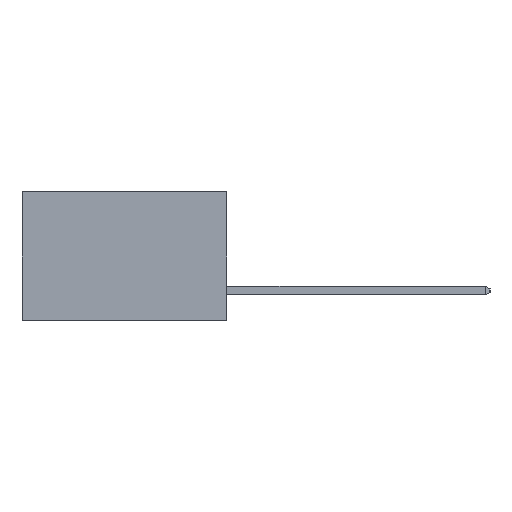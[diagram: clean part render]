
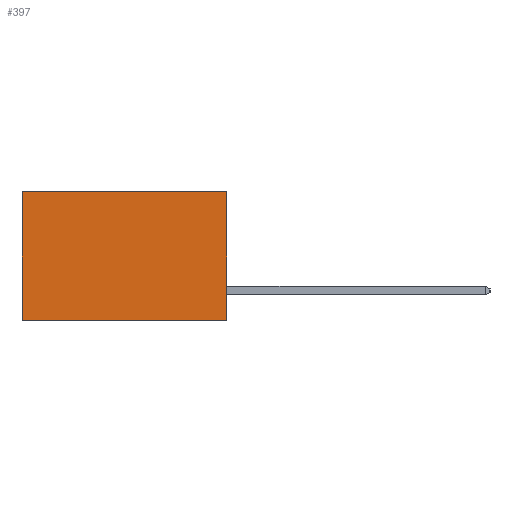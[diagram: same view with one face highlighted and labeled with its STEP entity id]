
A CAD part, left-side view. The second image highlights one B-rep face of the part: STEP entity #397.
In plain terms, the highlighted planar face has unit normal (-1, 0, 0).
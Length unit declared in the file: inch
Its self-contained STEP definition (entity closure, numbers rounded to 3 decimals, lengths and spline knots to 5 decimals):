
#125 = DIRECTION ( 'NONE',  ( 1., 0., 0. ) ) ;
#236 = PLANE ( 'NONE',  #12208 ) ;
#397 = ADVANCED_FACE ( 'NONE', ( #10097 ), #236, .F. ) ;
#1538 = LINE ( 'NONE', #20694, #6214 ) ;
#2117 = VERTEX_POINT ( 'NONE', #7028 ) ;
#2298 = DIRECTION ( 'NONE',  ( 0., 1., 0. ) ) ;
#2622 = EDGE_CURVE ( 'NONE', #4430, #13952, #1538, .T. ) ;
#3265 = LINE ( 'NONE', #6473, #20419 ) ;
#3658 = LINE ( 'NONE', #16107, #16915 ) ;
#4401 = VECTOR ( 'NONE', #17243, 39.37008 ) ;
#4430 = VERTEX_POINT ( 'NONE', #7166 ) ;
#6063 = ORIENTED_EDGE ( 'NONE', *, *, #21533, .T. ) ;
#6214 = VECTOR ( 'NONE', #10809, 39.37008 ) ;
#6473 = CARTESIAN_POINT ( 'NONE',  ( 0.277, 0.59, -0.37 ) ) ;
#6609 = ORIENTED_EDGE ( 'NONE', *, *, #15103, .F. ) ;
#7028 = CARTESIAN_POINT ( 'NONE',  ( 0.277, 0.59, 0. ) ) ;
#7159 = ORIENTED_EDGE ( 'NONE', *, *, #15989, .T. ) ;
#7166 = CARTESIAN_POINT ( 'NONE',  ( 0.277, 0., -0.37 ) ) ;
#7562 = CARTESIAN_POINT ( 'NONE',  ( 0.277, 0., 0. ) ) ;
#9679 = CARTESIAN_POINT ( 'NONE',  ( 0.277, 0., -0.37 ) ) ;
#10097 = FACE_OUTER_BOUND ( 'NONE', #11099, .T. ) ;
#10412 = DIRECTION ( 'NONE',  ( 0., 0., -1. ) ) ;
#10687 = ORIENTED_EDGE ( 'NONE', *, *, #2622, .F. ) ;
#10809 = DIRECTION ( 'NONE',  ( 0., 1., 0. ) ) ;
#11099 = EDGE_LOOP ( 'NONE', ( #6063, #10687, #6609, #7159 ) ) ;
#12208 = AXIS2_PLACEMENT_3D ( 'NONE', #9679, #125, #10412 ) ;
#13952 = VERTEX_POINT ( 'NONE', #21397 ) ;
#15103 = EDGE_CURVE ( 'NONE', #21789, #4430, #18675, .T. ) ;
#15535 = CARTESIAN_POINT ( 'NONE',  ( 0.277, 0., -0.37 ) ) ;
#15989 = EDGE_CURVE ( 'NONE', #21789, #2117, #3658, .T. ) ;
#16107 = CARTESIAN_POINT ( 'NONE',  ( 0.277, 0., 0. ) ) ;
#16915 = VECTOR ( 'NONE', #2298, 39.37008 ) ;
#17243 = DIRECTION ( 'NONE',  ( 0., 0., -1. ) ) ;
#18675 = LINE ( 'NONE', #15535, #4401 ) ;
#20129 = DIRECTION ( 'NONE',  ( 0., 0., -1. ) ) ;
#20419 = VECTOR ( 'NONE', #20129, 39.37008 ) ;
#20694 = CARTESIAN_POINT ( 'NONE',  ( 0.277, 0., -0.37 ) ) ;
#21397 = CARTESIAN_POINT ( 'NONE',  ( 0.277, 0.59, -0.37 ) ) ;
#21533 = EDGE_CURVE ( 'NONE', #2117, #13952, #3265, .T. ) ;
#21789 = VERTEX_POINT ( 'NONE', #7562 ) ;
